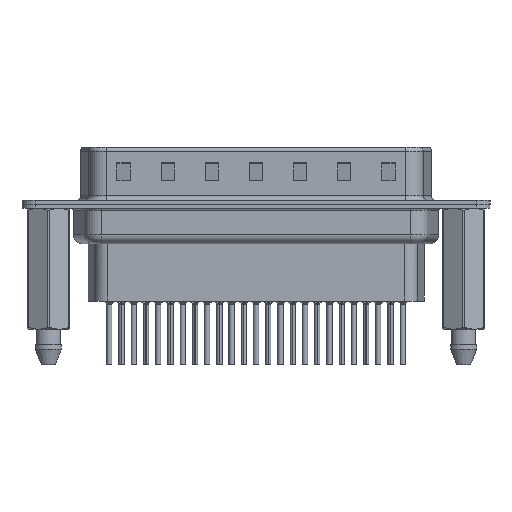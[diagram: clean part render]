
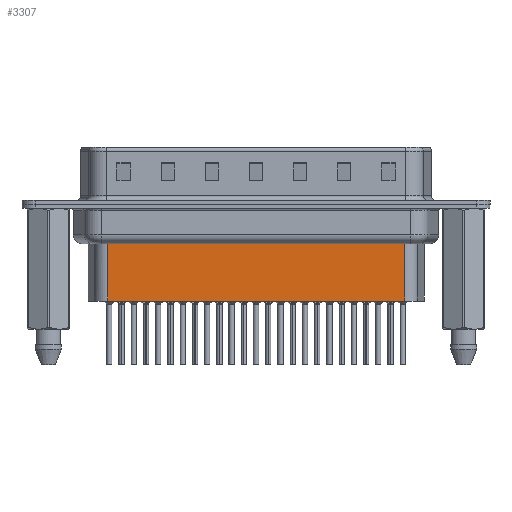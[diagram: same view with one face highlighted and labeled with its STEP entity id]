
A CAD part, front view. The second image highlights one B-rep face of the part: STEP entity #3307.
In plain terms, the highlighted planar face has unit normal (0, -1, 0).
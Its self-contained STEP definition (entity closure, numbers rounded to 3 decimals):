
#1007 = DIRECTION ( 'NONE',  ( -1., 0., 0. ) ) ;
#1221 = VECTOR ( 'NONE', #12725, 1000. ) ;
#1452 = CARTESIAN_POINT ( 'NONE',  ( 40.344, -3.5, -10.95 ) ) ;
#2560 = VERTEX_POINT ( 'NONE', #1452 ) ;
#2748 = VECTOR ( 'NONE', #5599, 1000. ) ;
#3307 = ADVANCED_FACE ( 'NONE', ( #16838 ), #3871, .T. ) ;
#3682 = VERTEX_POINT ( 'NONE', #4139 ) ;
#3871 = PLANE ( 'NONE',  #24136 ) ;
#4139 = CARTESIAN_POINT ( 'NONE',  ( 40.344, -3.5, -4.097 ) ) ;
#5118 = LINE ( 'NONE', #13718, #12004 ) ;
#5599 = DIRECTION ( 'NONE',  ( -1., 0., 0. ) ) ;
#7356 = ORIENTED_EDGE ( 'NONE', *, *, #13602, .T. ) ;
#7487 = CARTESIAN_POINT ( 'NONE',  ( 6.706, -3.5, -10.95 ) ) ;
#7636 = EDGE_CURVE ( 'NONE', #3682, #2560, #25528, .T. ) ;
#10252 = LINE ( 'NONE', #24893, #2748 ) ;
#12004 = VECTOR ( 'NONE', #22299, 1000. ) ;
#12347 = VECTOR ( 'NONE', #1007, 1000. ) ;
#12584 = VERTEX_POINT ( 'NONE', #26125 ) ;
#12618 = CARTESIAN_POINT ( 'NONE',  ( 6.706, -3.5, -3.1 ) ) ;
#12725 = DIRECTION ( 'NONE',  ( 0., 0., -1. ) ) ;
#13602 = EDGE_CURVE ( 'NONE', #3682, #25980, #10252, .T. ) ;
#13718 = CARTESIAN_POINT ( 'NONE',  ( 6.706, -3.5, -3.1 ) ) ;
#14118 = LINE ( 'NONE', #7487, #12347 ) ;
#14441 = CARTESIAN_POINT ( 'NONE',  ( 40.344, -3.5, -3.1 ) ) ;
#14768 = ORIENTED_EDGE ( 'NONE', *, *, #27736, .F. ) ;
#16394 = CARTESIAN_POINT ( 'NONE',  ( 6.706, -3.5, -4.097 ) ) ;
#16423 = DIRECTION ( 'NONE',  ( 0., -1., 0. ) ) ;
#16838 = FACE_OUTER_BOUND ( 'NONE', #23124, .T. ) ;
#18960 = DIRECTION ( 'NONE',  ( 1., 0., 0. ) ) ;
#19138 = ORIENTED_EDGE ( 'NONE', *, *, #21398, .T. ) ;
#21398 = EDGE_CURVE ( 'NONE', #25980, #12584, #5118, .T. ) ;
#22299 = DIRECTION ( 'NONE',  ( 0., 0., -1. ) ) ;
#23124 = EDGE_LOOP ( 'NONE', ( #24153, #7356, #19138, #14768 ) ) ;
#24136 = AXIS2_PLACEMENT_3D ( 'NONE', #12618, #16423, #18960 ) ;
#24153 = ORIENTED_EDGE ( 'NONE', *, *, #7636, .F. ) ;
#24893 = CARTESIAN_POINT ( 'NONE',  ( 6.459, -3.5, -4.097 ) ) ;
#25528 = LINE ( 'NONE', #14441, #1221 ) ;
#25980 = VERTEX_POINT ( 'NONE', #16394 ) ;
#26125 = CARTESIAN_POINT ( 'NONE',  ( 6.706, -3.5, -10.95 ) ) ;
#27736 = EDGE_CURVE ( 'NONE', #2560, #12584, #14118, .T. ) ;
